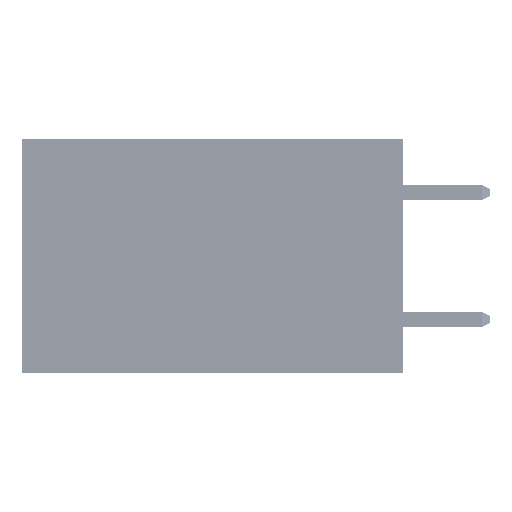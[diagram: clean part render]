
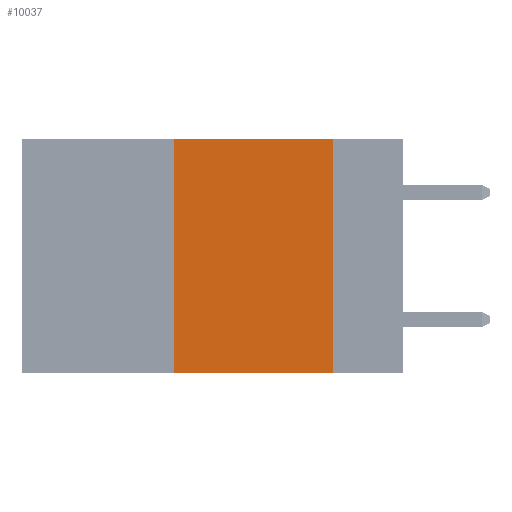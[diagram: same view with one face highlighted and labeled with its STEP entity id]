
A CAD part, left-side view. The second image highlights one B-rep face of the part: STEP entity #10037.
In plain terms, the highlighted planar face has unit normal (-1, 0, 0).
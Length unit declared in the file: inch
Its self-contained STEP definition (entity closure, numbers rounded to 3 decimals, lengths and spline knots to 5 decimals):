
#1988 = VECTOR ( 'NONE', #4583, 39.37008 ) ;
#4583 = DIRECTION ( 'NONE',  ( 0., 0., -1. ) ) ;
#5182 = EDGE_CURVE ( 'NONE', #18104, #25471, #13057, .T. ) ;
#9072 = ORIENTED_EDGE ( 'NONE', *, *, #5182, .F. ) ;
#10037 = ADVANCED_FACE ( 'NONE', ( #14451 ), #34595, .F. ) ;
#11011 = VERTEX_POINT ( 'NONE', #40172 ) ;
#11573 = AXIS2_PLACEMENT_3D ( 'NONE', #42648, #43002, #17939 ) ;
#13057 = LINE ( 'NONE', #50473, #1988 ) ;
#13647 = LINE ( 'NONE', #28615, #18805 ) ;
#14040 = CARTESIAN_POINT ( 'NONE',  ( 0., 0.11, -0.37 ) ) ;
#14451 = FACE_OUTER_BOUND ( 'NONE', #43732, .T. ) ;
#16053 = DIRECTION ( 'NONE',  ( 0., -1., 0. ) ) ;
#17508 = CARTESIAN_POINT ( 'NONE',  ( 0., 0.36, 0. ) ) ;
#17939 = DIRECTION ( 'NONE',  ( 0., 0., -1. ) ) ;
#18104 = VERTEX_POINT ( 'NONE', #42005 ) ;
#18805 = VECTOR ( 'NONE', #44998, 39.37008 ) ;
#20180 = EDGE_CURVE ( 'NONE', #47272, #18104, #49734, .T. ) ;
#25471 = VERTEX_POINT ( 'NONE', #14040 ) ;
#28362 = CARTESIAN_POINT ( 'NONE',  ( 0., 0.6, 0. ) ) ;
#28370 = VECTOR ( 'NONE', #38680, 39.37008 ) ;
#28615 = CARTESIAN_POINT ( 'NONE',  ( 0., 0.6, -0.37 ) ) ;
#34595 = PLANE ( 'NONE',  #11573 ) ;
#35474 = LINE ( 'NONE', #46848, #28370 ) ;
#37513 = ORIENTED_EDGE ( 'NONE', *, *, #46901, .F. ) ;
#38680 = DIRECTION ( 'NONE',  ( 0., 0., 1. ) ) ;
#39374 = VECTOR ( 'NONE', #16053, 39.37008 ) ;
#39621 = ORIENTED_EDGE ( 'NONE', *, *, #20180, .F. ) ;
#39658 = EDGE_CURVE ( 'NONE', #11011, #25471, #13647, .T. ) ;
#40172 = CARTESIAN_POINT ( 'NONE',  ( 0., 0.36, -0.37 ) ) ;
#41633 = ORIENTED_EDGE ( 'NONE', *, *, #39658, .T. ) ;
#42005 = CARTESIAN_POINT ( 'NONE',  ( 0., 0.11, 0. ) ) ;
#42648 = CARTESIAN_POINT ( 'NONE',  ( 0., 0.6, 0. ) ) ;
#43002 = DIRECTION ( 'NONE',  ( 1., 0., 0. ) ) ;
#43732 = EDGE_LOOP ( 'NONE', ( #9072, #39621, #37513, #41633 ) ) ;
#44998 = DIRECTION ( 'NONE',  ( 0., -1., 0. ) ) ;
#46848 = CARTESIAN_POINT ( 'NONE',  ( 0., 0.36, 0. ) ) ;
#46901 = EDGE_CURVE ( 'NONE', #11011, #47272, #35474, .T. ) ;
#47272 = VERTEX_POINT ( 'NONE', #17508 ) ;
#49734 = LINE ( 'NONE', #28362, #39374 ) ;
#50473 = CARTESIAN_POINT ( 'NONE',  ( 0., 0.11, 0. ) ) ;
